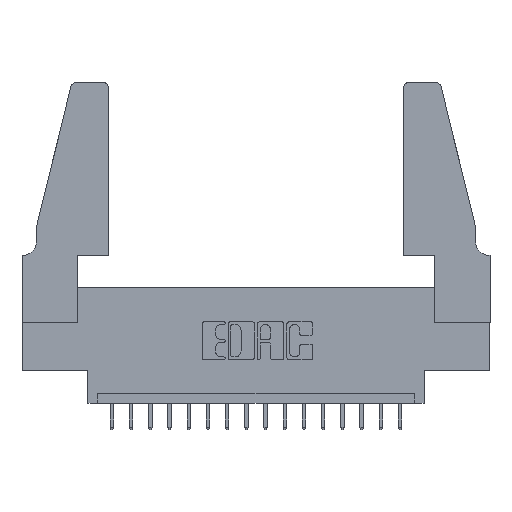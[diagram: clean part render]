
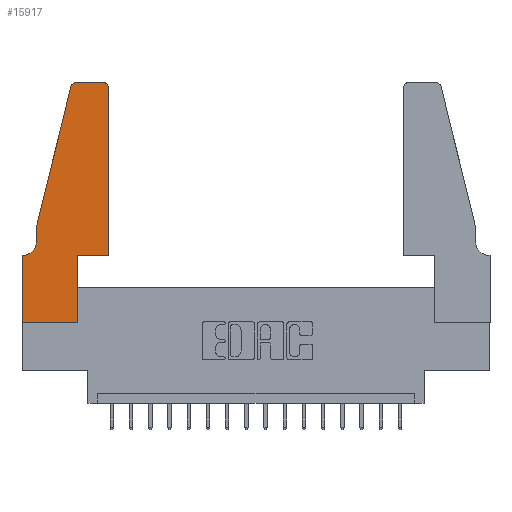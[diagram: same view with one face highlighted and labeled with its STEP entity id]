
A CAD part, top view. The second image highlights one B-rep face of the part: STEP entity #15917.
In plain terms, the highlighted planar face has unit normal (0, 0, 1).
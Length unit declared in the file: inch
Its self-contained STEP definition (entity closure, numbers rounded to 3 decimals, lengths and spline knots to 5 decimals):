
#203 = CARTESIAN_POINT ( 'NONE',  ( 0., 0., 0.37 ) ) ;
#284 = DIRECTION ( 'NONE',  ( 1., 0., 0. ) ) ;
#565 = VERTEX_POINT ( 'NONE', #1926 ) ;
#867 = ORIENTED_EDGE ( 'NONE', *, *, #4065, .T. ) ;
#974 = DIRECTION ( 'NONE',  ( 0., 0., 1. ) ) ;
#1137 = CARTESIAN_POINT ( 'NONE',  ( 0.2865, 0.35, 0.37 ) ) ;
#1491 = CARTESIAN_POINT ( 'NONE',  ( 0.4205, 1.25, 0.37 ) ) ;
#1520 = DIRECTION ( 'NONE',  ( -1., 0., 0. ) ) ;
#1604 = CARTESIAN_POINT ( 'NONE',  ( 0.0755, 0.35, 0.37 ) ) ;
#1609 = VERTEX_POINT ( 'NONE', #7163 ) ;
#1782 = DIRECTION ( 'NONE',  ( -0.239, -0.971, 0. ) ) ;
#1817 = VERTEX_POINT ( 'NONE', #1491 ) ;
#1824 = VECTOR ( 'NONE', #1782, 39.37008 ) ;
#1926 = CARTESIAN_POINT ( 'NONE',  ( 0.284, 1.25, 0.37 ) ) ;
#1934 = LINE ( 'NONE', #10239, #15128 ) ;
#2050 = DIRECTION ( 'NONE',  ( 0., -1., 0. ) ) ;
#2199 = VERTEX_POINT ( 'NONE', #7480 ) ;
#2709 = ORIENTED_EDGE ( 'NONE', *, *, #14238, .T. ) ;
#3341 = VECTOR ( 'NONE', #9441, 39.37008 ) ;
#4065 = EDGE_CURVE ( 'NONE', #10837, #1817, #9752, .T. ) ;
#4327 = AXIS2_PLACEMENT_3D ( 'NONE', #6131, #11649, #14468 ) ;
#4671 = CARTESIAN_POINT ( 'NONE',  ( 0.2865, 0.35, 0.37 ) ) ;
#4758 = DIRECTION ( 'NONE',  ( 0., 1., 0. ) ) ;
#4812 = ORIENTED_EDGE ( 'NONE', *, *, #10879, .T. ) ;
#5092 = DIRECTION ( 'NONE',  ( 1., 0., 0. ) ) ;
#5170 = AXIS2_PLACEMENT_3D ( 'NONE', #12766, #16627, #284 ) ;
#5598 = DIRECTION ( 'NONE',  ( 1., 0., 0. ) ) ;
#6131 = CARTESIAN_POINT ( 'NONE',  ( 0.0055, 0.42, 0.37 ) ) ;
#6399 = CIRCLE ( 'NONE', #4327, 0.07 ) ;
#6537 = DIRECTION ( 'NONE',  ( 1., 0., 0. ) ) ;
#6675 = EDGE_CURVE ( 'NONE', #1609, #14704, #13844, .T. ) ;
#6734 = VERTEX_POINT ( 'NONE', #203 ) ;
#7058 = CARTESIAN_POINT ( 'NONE',  ( 0.4505, 1.22, 0.37 ) ) ;
#7112 = CARTESIAN_POINT ( 'NONE',  ( 0.4505, 0.35, 0.37 ) ) ;
#7163 = CARTESIAN_POINT ( 'NONE',  ( 0.0755, 0.5, 0.37 ) ) ;
#7166 = LINE ( 'NONE', #15683, #1824 ) ;
#7227 = EDGE_CURVE ( 'NONE', #1817, #565, #1934, .T. ) ;
#7241 = DIRECTION ( 'NONE',  ( 1., 0., 0. ) ) ;
#7479 = DIRECTION ( 'NONE',  ( 0., 0., 1. ) ) ;
#7480 = CARTESIAN_POINT ( 'NONE',  ( 0.2865, 0., 0.37 ) ) ;
#7695 = ORIENTED_EDGE ( 'NONE', *, *, #9459, .T. ) ;
#7780 = EDGE_CURVE ( 'NONE', #17871, #12543, #8700, .T. ) ;
#8558 = ORIENTED_EDGE ( 'NONE', *, *, #7227, .T. ) ;
#8700 = LINE ( 'NONE', #12698, #17183 ) ;
#8760 = ORIENTED_EDGE ( 'NONE', *, *, #12202, .T. ) ;
#9081 = LINE ( 'NONE', #14485, #11754 ) ;
#9436 = CARTESIAN_POINT ( 'NONE',  ( 0., 0.35, 0.37 ) ) ;
#9441 = DIRECTION ( 'NONE',  ( 0., 1., 0. ) ) ;
#9459 = EDGE_CURVE ( 'NONE', #9843, #1609, #7166, .T. ) ;
#9752 = CIRCLE ( 'NONE', #15286, 0.03 ) ;
#9805 = CIRCLE ( 'NONE', #17285, 0.03 ) ;
#9843 = VERTEX_POINT ( 'NONE', #15569 ) ;
#9885 = PLANE ( 'NONE',  #5170 ) ;
#10239 = CARTESIAN_POINT ( 'NONE',  ( 0.2605, 1.25, 0.37 ) ) ;
#10366 = ORIENTED_EDGE ( 'NONE', *, *, #17778, .T. ) ;
#10494 = ORIENTED_EDGE ( 'NONE', *, *, #11484, .T. ) ;
#10786 = CARTESIAN_POINT ( 'NONE',  ( 0.0755, 0.5, 0.37 ) ) ;
#10837 = VERTEX_POINT ( 'NONE', #7058 ) ;
#10879 = EDGE_CURVE ( 'NONE', #15208, #6734, #9081, .T. ) ;
#10941 = VERTEX_POINT ( 'NONE', #17099 ) ;
#11483 = DIRECTION ( 'NONE',  ( -1., 0., 0. ) ) ;
#11484 = EDGE_CURVE ( 'NONE', #2199, #17871, #13582, .T. ) ;
#11649 = DIRECTION ( 'NONE',  ( 0., 0., -1. ) ) ;
#11668 = VECTOR ( 'NONE', #16268, 39.37008 ) ;
#11754 = VECTOR ( 'NONE', #2050, 39.37008 ) ;
#12146 = VECTOR ( 'NONE', #1520, 39.37008 ) ;
#12202 = EDGE_CURVE ( 'NONE', #12543, #10837, #14216, .T. ) ;
#12430 = CARTESIAN_POINT ( 'NONE',  ( 0., 0., 0.37 ) ) ;
#12543 = VERTEX_POINT ( 'NONE', #7112 ) ;
#12585 = FACE_OUTER_BOUND ( 'NONE', #14454, .T. ) ;
#12698 = CARTESIAN_POINT ( 'NONE',  ( 0.4505, 0.35, 0.37 ) ) ;
#12766 = CARTESIAN_POINT ( 'NONE',  ( 0., 0.35, 0.37 ) ) ;
#13378 = CARTESIAN_POINT ( 'NONE',  ( 0.0755, 0.42, 0.37 ) ) ;
#13437 = CARTESIAN_POINT ( 'NONE',  ( 0.4205, 1.22, 0.37 ) ) ;
#13582 = LINE ( 'NONE', #1137, #3341 ) ;
#13844 = LINE ( 'NONE', #10786, #11668 ) ;
#14036 = LINE ( 'NONE', #12430, #15258 ) ;
#14054 = LINE ( 'NONE', #1604, #12146 ) ;
#14216 = LINE ( 'NONE', #14399, #17276 ) ;
#14238 = EDGE_CURVE ( 'NONE', #565, #9843, #9805, .T. ) ;
#14399 = CARTESIAN_POINT ( 'NONE',  ( 0.4505, 0.35, 0.37 ) ) ;
#14454 = EDGE_LOOP ( 'NONE', ( #8558, #2709, #7695, #16091, #10366, #15191, #4812, #17789, #10494, #16269, #8760, #867 ) ) ;
#14468 = DIRECTION ( 'NONE',  ( -1., 0., 0. ) ) ;
#14485 = CARTESIAN_POINT ( 'NONE',  ( 0., 0., 0.37 ) ) ;
#14704 = VERTEX_POINT ( 'NONE', #13378 ) ;
#14759 = EDGE_CURVE ( 'NONE', #6734, #2199, #14036, .T. ) ;
#15128 = VECTOR ( 'NONE', #11483, 39.37008 ) ;
#15191 = ORIENTED_EDGE ( 'NONE', *, *, #16364, .T. ) ;
#15208 = VERTEX_POINT ( 'NONE', #9436 ) ;
#15258 = VECTOR ( 'NONE', #5598, 39.37008 ) ;
#15286 = AXIS2_PLACEMENT_3D ( 'NONE', #13437, #974, #6537 ) ;
#15569 = CARTESIAN_POINT ( 'NONE',  ( 0.25487, 1.22718, 0.37 ) ) ;
#15683 = CARTESIAN_POINT ( 'NONE',  ( 0.0755, 0.5, 0.37 ) ) ;
#15917 = ADVANCED_FACE ( 'NONE', ( #12585 ), #9885, .T. ) ;
#16091 = ORIENTED_EDGE ( 'NONE', *, *, #6675, .T. ) ;
#16268 = DIRECTION ( 'NONE',  ( 0., -1., 0. ) ) ;
#16269 = ORIENTED_EDGE ( 'NONE', *, *, #7780, .T. ) ;
#16364 = EDGE_CURVE ( 'NONE', #10941, #15208, #14054, .T. ) ;
#16627 = DIRECTION ( 'NONE',  ( 0., 0., 1. ) ) ;
#17099 = CARTESIAN_POINT ( 'NONE',  ( 0.0055, 0.35, 0.37 ) ) ;
#17183 = VECTOR ( 'NONE', #7241, 39.37008 ) ;
#17245 = CARTESIAN_POINT ( 'NONE',  ( 0.284, 1.22, 0.37 ) ) ;
#17276 = VECTOR ( 'NONE', #4758, 39.37008 ) ;
#17285 = AXIS2_PLACEMENT_3D ( 'NONE', #17245, #7479, #5092 ) ;
#17778 = EDGE_CURVE ( 'NONE', #14704, #10941, #6399, .T. ) ;
#17789 = ORIENTED_EDGE ( 'NONE', *, *, #14759, .T. ) ;
#17871 = VERTEX_POINT ( 'NONE', #4671 ) ;
